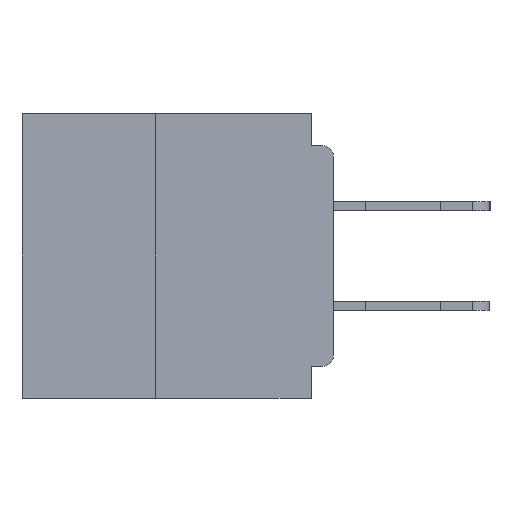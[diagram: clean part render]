
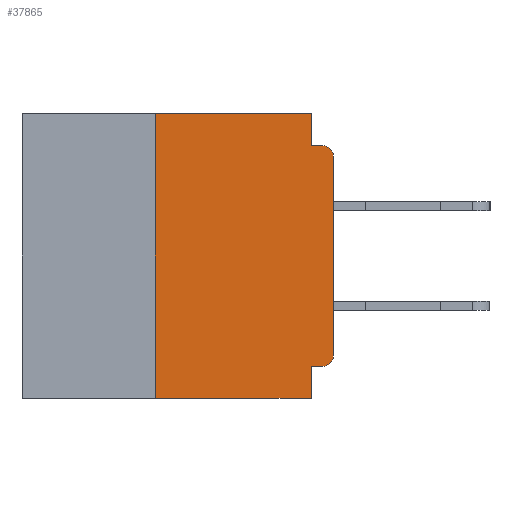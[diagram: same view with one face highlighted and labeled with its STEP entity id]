
A CAD part, left-side view. The second image highlights one B-rep face of the part: STEP entity #37865.
In plain terms, the highlighted planar face has unit normal (-1, 0, 0).
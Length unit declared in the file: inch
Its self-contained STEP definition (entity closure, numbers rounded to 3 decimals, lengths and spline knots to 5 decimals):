
#63 = CARTESIAN_POINT ( 'NONE',  ( 0., 0., -0.045 ) ) ;
#854 = VERTEX_POINT ( 'NONE', #17317 ) ;
#1059 = DIRECTION ( 'NONE',  ( 0., 0., -1. ) ) ;
#1504 = EDGE_CURVE ( 'NONE', #25968, #854, #12160, .T. ) ;
#2125 = VECTOR ( 'NONE', #5577, 39.37008 ) ;
#2397 = CARTESIAN_POINT ( 'NONE',  ( 0., 0., -0.355 ) ) ;
#2493 = EDGE_CURVE ( 'NONE', #854, #4469, #47376, .T. ) ;
#3596 = DIRECTION ( 'NONE',  ( 0., 0., -1. ) ) ;
#4235 = VECTOR ( 'NONE', #26386, 39.37008 ) ;
#4469 = VERTEX_POINT ( 'NONE', #20741 ) ;
#4825 = CARTESIAN_POINT ( 'NONE',  ( 0., 0.25, 0. ) ) ;
#5577 = DIRECTION ( 'NONE',  ( 0., -1., 0. ) ) ;
#6035 = VERTEX_POINT ( 'NONE', #33490 ) ;
#6191 = DIRECTION ( 'NONE',  ( 0., 1., 0. ) ) ;
#6938 = CARTESIAN_POINT ( 'NONE',  ( 0., 0.015, -0.045 ) ) ;
#6983 = CARTESIAN_POINT ( 'NONE',  ( 0., 0.015, -0.06 ) ) ;
#7539 = DIRECTION ( 'NONE',  ( 0., 0., 1. ) ) ;
#7775 = ORIENTED_EDGE ( 'NONE', *, *, #37158, .F. ) ;
#9439 = ORIENTED_EDGE ( 'NONE', *, *, #41373, .T. ) ;
#10786 = DIRECTION ( 'NONE',  ( 0., 0., -1. ) ) ;
#12160 = LINE ( 'NONE', #24149, #2125 ) ;
#13566 = EDGE_CURVE ( 'NONE', #33202, #43350, #34376, .T. ) ;
#13697 = LINE ( 'NONE', #2397, #32508 ) ;
#14594 = CARTESIAN_POINT ( 'NONE',  ( 0., 0., -0.34 ) ) ;
#14605 = VERTEX_POINT ( 'NONE', #6938 ) ;
#15418 = AXIS2_PLACEMENT_3D ( 'NONE', #48686, #26129, #3596 ) ;
#15846 = CARTESIAN_POINT ( 'NONE',  ( 0., 0.437, 0. ) ) ;
#16248 = EDGE_CURVE ( 'NONE', #26216, #34696, #26961, .T. ) ;
#17317 = CARTESIAN_POINT ( 'NONE',  ( 0., 0.031, 0. ) ) ;
#17452 = EDGE_LOOP ( 'NONE', ( #20856, #26552, #20455, #19273, #30351, #28252, #46648, #7775, #25094, #9439 ) ) ;
#18690 = CARTESIAN_POINT ( 'NONE',  ( 0., 0., 0. ) ) ;
#19273 = ORIENTED_EDGE ( 'NONE', *, *, #2493, .F. ) ;
#20455 = ORIENTED_EDGE ( 'NONE', *, *, #32999, .F. ) ;
#20741 = CARTESIAN_POINT ( 'NONE',  ( 0., 0.031, -0.045 ) ) ;
#20856 = ORIENTED_EDGE ( 'NONE', *, *, #13566, .T. ) ;
#21574 = AXIS2_PLACEMENT_3D ( 'NONE', #15846, #23590, #1059 ) ;
#22910 = DIRECTION ( 'NONE',  ( 0., 0., -1. ) ) ;
#22939 = LINE ( 'NONE', #32440, #32978 ) ;
#23590 = DIRECTION ( 'NONE',  ( 1., 0., 0. ) ) ;
#24149 = CARTESIAN_POINT ( 'NONE',  ( 0., 0.437, 0. ) ) ;
#24342 = VECTOR ( 'NONE', #7539, 39.37008 ) ;
#25094 = ORIENTED_EDGE ( 'NONE', *, *, #32778, .F. ) ;
#25179 = CARTESIAN_POINT ( 'NONE',  ( 0., 0.25, -0.4 ) ) ;
#25678 = EDGE_CURVE ( 'NONE', #43350, #14605, #46822, .T. ) ;
#25741 = CIRCLE ( 'NONE', #15418, 0.015 ) ;
#25968 = VERTEX_POINT ( 'NONE', #4825 ) ;
#26129 = DIRECTION ( 'NONE',  ( -1., 0., 0. ) ) ;
#26216 = VERTEX_POINT ( 'NONE', #25179 ) ;
#26386 = DIRECTION ( 'NONE',  ( 0., -1., 0. ) ) ;
#26552 = ORIENTED_EDGE ( 'NONE', *, *, #25678, .T. ) ;
#26898 = CARTESIAN_POINT ( 'NONE',  ( 0., 0.031, 0. ) ) ;
#26961 = LINE ( 'NONE', #28753, #43482 ) ;
#27536 = AXIS2_PLACEMENT_3D ( 'NONE', #6983, #33309, #10786 ) ;
#28252 = ORIENTED_EDGE ( 'NONE', *, *, #28438, .F. ) ;
#28438 = EDGE_CURVE ( 'NONE', #26216, #25968, #22939, .T. ) ;
#28753 = CARTESIAN_POINT ( 'NONE',  ( 0., 0.437, -0.4 ) ) ;
#30351 = ORIENTED_EDGE ( 'NONE', *, *, #1504, .F. ) ;
#31030 = PLANE ( 'NONE',  #21574 ) ;
#31435 = CARTESIAN_POINT ( 'NONE',  ( 0., 0.031, -0.4 ) ) ;
#31814 = CARTESIAN_POINT ( 'NONE',  ( 0., 0.015, -0.355 ) ) ;
#32440 = CARTESIAN_POINT ( 'NONE',  ( 0., 0.25, -0.4 ) ) ;
#32508 = VECTOR ( 'NONE', #6191, 39.37008 ) ;
#32522 = DIRECTION ( 'NONE',  ( 0., -1., 0. ) ) ;
#32778 = EDGE_CURVE ( 'NONE', #34130, #6035, #13697, .T. ) ;
#32978 = VECTOR ( 'NONE', #40048, 39.37008 ) ;
#32999 = EDGE_CURVE ( 'NONE', #4469, #14605, #33080, .T. ) ;
#33080 = LINE ( 'NONE', #63, #4235 ) ;
#33202 = VERTEX_POINT ( 'NONE', #14594 ) ;
#33309 = DIRECTION ( 'NONE',  ( -1., 0., 0. ) ) ;
#33490 = CARTESIAN_POINT ( 'NONE',  ( 0., 0.031, -0.355 ) ) ;
#33781 = FACE_OUTER_BOUND ( 'NONE', #17452, .T. ) ;
#34130 = VERTEX_POINT ( 'NONE', #31814 ) ;
#34376 = LINE ( 'NONE', #18690, #24342 ) ;
#34529 = CARTESIAN_POINT ( 'NONE',  ( 0., 0.031, -0.4 ) ) ;
#34696 = VERTEX_POINT ( 'NONE', #31435 ) ;
#36867 = CARTESIAN_POINT ( 'NONE',  ( 0., 0., -0.06 ) ) ;
#37158 = EDGE_CURVE ( 'NONE', #6035, #34696, #46831, .T. ) ;
#37345 = VECTOR ( 'NONE', #22910, 39.37008 ) ;
#37865 = ADVANCED_FACE ( 'NONE', ( #33781 ), #31030, .F. ) ;
#38325 = DIRECTION ( 'NONE',  ( 0., 0., -1. ) ) ;
#40048 = DIRECTION ( 'NONE',  ( 0., 0., 1. ) ) ;
#41373 = EDGE_CURVE ( 'NONE', #34130, #33202, #25741, .T. ) ;
#43350 = VERTEX_POINT ( 'NONE', #36867 ) ;
#43482 = VECTOR ( 'NONE', #32522, 39.37008 ) ;
#44490 = VECTOR ( 'NONE', #38325, 39.37008 ) ;
#46648 = ORIENTED_EDGE ( 'NONE', *, *, #16248, .T. ) ;
#46822 = CIRCLE ( 'NONE', #27536, 0.015 ) ;
#46831 = LINE ( 'NONE', #34529, #44490 ) ;
#47376 = LINE ( 'NONE', #26898, #37345 ) ;
#48686 = CARTESIAN_POINT ( 'NONE',  ( 0., 0.015, -0.34 ) ) ;
